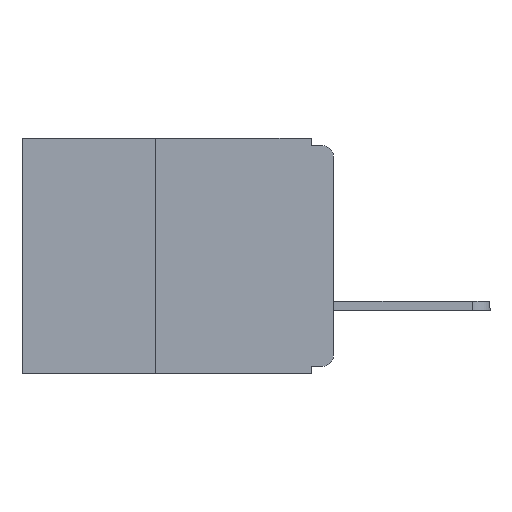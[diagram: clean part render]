
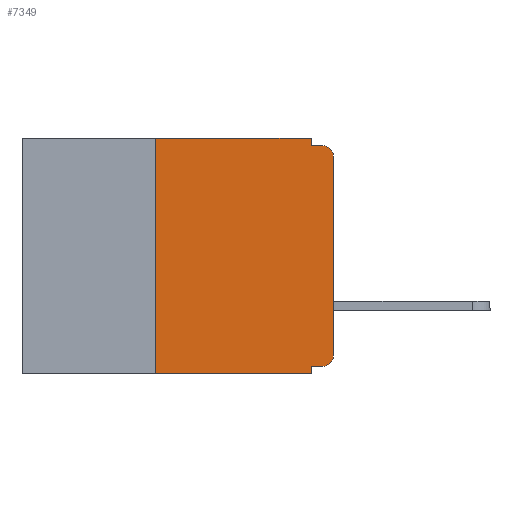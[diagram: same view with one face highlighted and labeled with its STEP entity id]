
A CAD part, left-side view. The second image highlights one B-rep face of the part: STEP entity #7349.
In plain terms, the highlighted planar face has unit normal (-1, 0, 0).
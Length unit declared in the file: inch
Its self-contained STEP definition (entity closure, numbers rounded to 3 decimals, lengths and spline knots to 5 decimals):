
#19 = ORIENTED_EDGE ( 'NONE', *, *, #11417, .T. ) ;
#180 = ORIENTED_EDGE ( 'NONE', *, *, #1876, .T. ) ;
#353 = ORIENTED_EDGE ( 'NONE', *, *, #6005, .F. ) ;
#518 = DIRECTION ( 'NONE',  ( 0., 0., 1. ) ) ;
#639 = EDGE_LOOP ( 'NONE', ( #19, #8155, #14268, #1374, #353, #668, #180, #2764, #15111, #3398 ) ) ;
#668 = ORIENTED_EDGE ( 'NONE', *, *, #1740, .F. ) ;
#769 = AXIS2_PLACEMENT_3D ( 'NONE', #8737, #8715, #8645 ) ;
#1374 = ORIENTED_EDGE ( 'NONE', *, *, #1702, .F. ) ;
#1686 = LINE ( 'NONE', #3381, #1937 ) ;
#1702 = EDGE_CURVE ( 'NONE', #8967, #13058, #2954, .T. ) ;
#1740 = EDGE_CURVE ( 'NONE', #2548, #13512, #2465, .T. ) ;
#1876 = EDGE_CURVE ( 'NONE', #2548, #14507, #1686, .T. ) ;
#1937 = VECTOR ( 'NONE', #3319, 39.37008 ) ;
#2465 = LINE ( 'NONE', #10321, #2497 ) ;
#2497 = VECTOR ( 'NONE', #518, 39.37008 ) ;
#2533 = VECTOR ( 'NONE', #16091, 39.37008 ) ;
#2548 = VERTEX_POINT ( 'NONE', #9767 ) ;
#2764 = ORIENTED_EDGE ( 'NONE', *, *, #10413, .F. ) ;
#2954 = LINE ( 'NONE', #15601, #2533 ) ;
#2972 = CARTESIAN_POINT ( 'NONE',  ( 0., 0.437, 0. ) ) ;
#3215 = DIRECTION ( 'NONE',  ( 0., -1., 0. ) ) ;
#3319 = DIRECTION ( 'NONE',  ( 0., -1., 0. ) ) ;
#3334 = LINE ( 'NONE', #13953, #3555 ) ;
#3381 = CARTESIAN_POINT ( 'NONE',  ( 0., 0.437, -0.33 ) ) ;
#3398 = ORIENTED_EDGE ( 'NONE', *, *, #9885, .T. ) ;
#3555 = VECTOR ( 'NONE', #13846, 39.37008 ) ;
#3842 = CARTESIAN_POINT ( 'NONE',  ( 0., 0., -0.305 ) ) ;
#4142 = DIRECTION ( 'NONE',  ( 0., 1., 0. ) ) ;
#4396 = CARTESIAN_POINT ( 'NONE',  ( 0., 0., -0.32 ) ) ;
#5175 = CIRCLE ( 'NONE', #11815, 0.015 ) ;
#5381 = VERTEX_POINT ( 'NONE', #3842 ) ;
#5437 = VECTOR ( 'NONE', #3215, 39.37008 ) ;
#5679 = VERTEX_POINT ( 'NONE', #7022 ) ;
#5856 = LINE ( 'NONE', #2972, #5437 ) ;
#6005 = EDGE_CURVE ( 'NONE', #13512, #8967, #5856, .T. ) ;
#6813 = CARTESIAN_POINT ( 'NONE',  ( 0., 0.031, 0. ) ) ;
#7022 = CARTESIAN_POINT ( 'NONE',  ( 0., 0.031, -0.32 ) ) ;
#7349 = ADVANCED_FACE ( 'NONE', ( #13043 ), #9800, .F. ) ;
#7509 = CARTESIAN_POINT ( 'NONE',  ( 0., 0.031, -0.33 ) ) ;
#7656 = VERTEX_POINT ( 'NONE', #10674 ) ;
#8006 = CIRCLE ( 'NONE', #769, 0.015 ) ;
#8155 = ORIENTED_EDGE ( 'NONE', *, *, #15291, .T. ) ;
#8645 = DIRECTION ( 'NONE',  ( 0., 0., -1. ) ) ;
#8715 = DIRECTION ( 'NONE',  ( -1., 0., 0. ) ) ;
#8726 = EDGE_CURVE ( 'NONE', #13058, #11471, #8946, .T. ) ;
#8737 = CARTESIAN_POINT ( 'NONE',  ( 0., 0.015, -0.025 ) ) ;
#8873 = VECTOR ( 'NONE', #16068, 39.37008 ) ;
#8946 = LINE ( 'NONE', #16308, #8873 ) ;
#8967 = VERTEX_POINT ( 'NONE', #6813 ) ;
#9627 = CARTESIAN_POINT ( 'NONE',  ( 0., 0.031, -0.01 ) ) ;
#9684 = DIRECTION ( 'NONE',  ( 0., 0., -1. ) ) ;
#9714 = DIRECTION ( 'NONE',  ( 1., 0., 0. ) ) ;
#9767 = CARTESIAN_POINT ( 'NONE',  ( 0., 0.25, -0.33 ) ) ;
#9800 = PLANE ( 'NONE',  #14307 ) ;
#9842 = CARTESIAN_POINT ( 'NONE',  ( 0., 0.437, 0. ) ) ;
#9885 = EDGE_CURVE ( 'NONE', #13860, #5381, #5175, .T. ) ;
#10321 = CARTESIAN_POINT ( 'NONE',  ( 0., 0.25, -0.33 ) ) ;
#10413 = EDGE_CURVE ( 'NONE', #5679, #14507, #3334, .T. ) ;
#10674 = CARTESIAN_POINT ( 'NONE',  ( 0., 0., -0.025 ) ) ;
#10978 = LINE ( 'NONE', #4396, #10993 ) ;
#10993 = VECTOR ( 'NONE', #4142, 39.37008 ) ;
#11417 = EDGE_CURVE ( 'NONE', #5381, #7656, #15788, .T. ) ;
#11471 = VERTEX_POINT ( 'NONE', #14299 ) ;
#11815 = AXIS2_PLACEMENT_3D ( 'NONE', #15014, #14925, #14642 ) ;
#13009 = CARTESIAN_POINT ( 'NONE',  ( 0., 0.015, -0.32 ) ) ;
#13043 = FACE_OUTER_BOUND ( 'NONE', #639, .T. ) ;
#13058 = VERTEX_POINT ( 'NONE', #9627 ) ;
#13512 = VERTEX_POINT ( 'NONE', #16258 ) ;
#13846 = DIRECTION ( 'NONE',  ( 0., 0., -1. ) ) ;
#13860 = VERTEX_POINT ( 'NONE', #13009 ) ;
#13953 = CARTESIAN_POINT ( 'NONE',  ( 0., 0.031, -0.33 ) ) ;
#14268 = ORIENTED_EDGE ( 'NONE', *, *, #8726, .F. ) ;
#14299 = CARTESIAN_POINT ( 'NONE',  ( 0., 0.015, -0.01 ) ) ;
#14307 = AXIS2_PLACEMENT_3D ( 'NONE', #9842, #9714, #9684 ) ;
#14382 = EDGE_CURVE ( 'NONE', #13860, #5679, #10978, .T. ) ;
#14507 = VERTEX_POINT ( 'NONE', #7509 ) ;
#14642 = DIRECTION ( 'NONE',  ( 0., 0., -1. ) ) ;
#14925 = DIRECTION ( 'NONE',  ( -1., 0., 0. ) ) ;
#15014 = CARTESIAN_POINT ( 'NONE',  ( 0., 0.015, -0.305 ) ) ;
#15111 = ORIENTED_EDGE ( 'NONE', *, *, #14382, .F. ) ;
#15291 = EDGE_CURVE ( 'NONE', #7656, #11471, #8006, .T. ) ;
#15307 = DIRECTION ( 'NONE',  ( 0., 0., 1. ) ) ;
#15466 = CARTESIAN_POINT ( 'NONE',  ( 0., 0., 0. ) ) ;
#15601 = CARTESIAN_POINT ( 'NONE',  ( 0., 0.031, 0. ) ) ;
#15788 = LINE ( 'NONE', #15466, #17012 ) ;
#16068 = DIRECTION ( 'NONE',  ( 0., -1., 0. ) ) ;
#16091 = DIRECTION ( 'NONE',  ( 0., 0., -1. ) ) ;
#16258 = CARTESIAN_POINT ( 'NONE',  ( 0., 0.25, 0. ) ) ;
#16308 = CARTESIAN_POINT ( 'NONE',  ( 0., 0., -0.01 ) ) ;
#17012 = VECTOR ( 'NONE', #15307, 39.37008 ) ;
